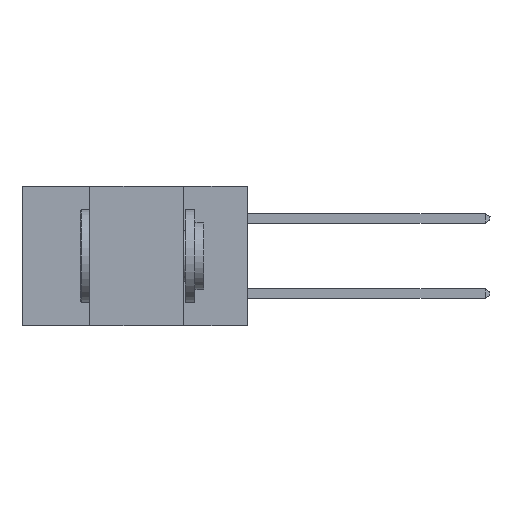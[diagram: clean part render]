
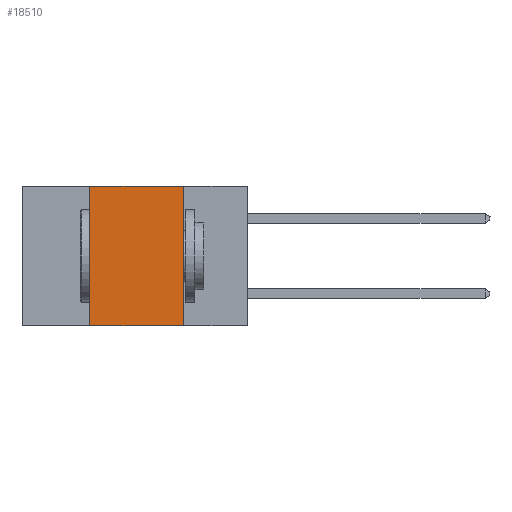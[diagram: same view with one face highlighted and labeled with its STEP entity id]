
A CAD part, left-side view. The second image highlights one B-rep face of the part: STEP entity #18510.
In plain terms, the highlighted planar face has unit normal (-1, 0, 0).
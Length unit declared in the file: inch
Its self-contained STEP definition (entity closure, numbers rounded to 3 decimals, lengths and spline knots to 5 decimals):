
#347 = DIRECTION ( 'NONE',  ( 0., 0., -1. ) ) ;
#397 = CARTESIAN_POINT ( 'NONE',  ( 0., 0.42, 0. ) ) ;
#1541 = CARTESIAN_POINT ( 'NONE',  ( 0., 0.6, 0. ) ) ;
#5013 = EDGE_CURVE ( 'NONE', #6420, #5768, #17414, .T. ) ;
#5149 = CARTESIAN_POINT ( 'NONE',  ( 0., 0.6, -0.37 ) ) ;
#5768 = VERTEX_POINT ( 'NONE', #10495 ) ;
#6420 = VERTEX_POINT ( 'NONE', #13045 ) ;
#6592 = VECTOR ( 'NONE', #14342, 39.37008 ) ;
#6649 = LINE ( 'NONE', #7069, #14434 ) ;
#6750 = AXIS2_PLACEMENT_3D ( 'NONE', #18619, #15017, #9464 ) ;
#7069 = CARTESIAN_POINT ( 'NONE',  ( 0., 0.42, 0. ) ) ;
#7657 = EDGE_LOOP ( 'NONE', ( #18190, #15180, #10925, #10163 ) ) ;
#7943 = VECTOR ( 'NONE', #347, 39.37008 ) ;
#8070 = EDGE_CURVE ( 'NONE', #8233, #6420, #17791, .T. ) ;
#8233 = VERTEX_POINT ( 'NONE', #397 ) ;
#8934 = DIRECTION ( 'NONE',  ( 0., -1., 0. ) ) ;
#9138 = CARTESIAN_POINT ( 'NONE',  ( 0., 0.17, 0. ) ) ;
#9464 = DIRECTION ( 'NONE',  ( 0., 0., -1. ) ) ;
#10163 = ORIENTED_EDGE ( 'NONE', *, *, #19307, .T. ) ;
#10495 = CARTESIAN_POINT ( 'NONE',  ( 0., 0.17, -0.37 ) ) ;
#10925 = ORIENTED_EDGE ( 'NONE', *, *, #16846, .F. ) ;
#13045 = CARTESIAN_POINT ( 'NONE',  ( 0., 0.17, 0. ) ) ;
#13160 = PLANE ( 'NONE',  #6750 ) ;
#14342 = DIRECTION ( 'NONE',  ( 0., -1., 0. ) ) ;
#14434 = VECTOR ( 'NONE', #16302, 39.37008 ) ;
#15017 = DIRECTION ( 'NONE',  ( 1., 0., 0. ) ) ;
#15180 = ORIENTED_EDGE ( 'NONE', *, *, #8070, .F. ) ;
#16302 = DIRECTION ( 'NONE',  ( 0., 0., 1. ) ) ;
#16846 = EDGE_CURVE ( 'NONE', #17405, #8233, #6649, .T. ) ;
#17405 = VERTEX_POINT ( 'NONE', #18946 ) ;
#17414 = LINE ( 'NONE', #9138, #7943 ) ;
#17791 = LINE ( 'NONE', #1541, #6592 ) ;
#18190 = ORIENTED_EDGE ( 'NONE', *, *, #5013, .F. ) ;
#18510 = ADVANCED_FACE ( 'NONE', ( #20942 ), #13160, .F. ) ;
#18619 = CARTESIAN_POINT ( 'NONE',  ( 0., 0.6, 0. ) ) ;
#18946 = CARTESIAN_POINT ( 'NONE',  ( 0., 0.42, -0.37 ) ) ;
#19307 = EDGE_CURVE ( 'NONE', #17405, #5768, #22465, .T. ) ;
#20942 = FACE_OUTER_BOUND ( 'NONE', #7657, .T. ) ;
#21037 = VECTOR ( 'NONE', #8934, 39.37008 ) ;
#22465 = LINE ( 'NONE', #5149, #21037 ) ;
